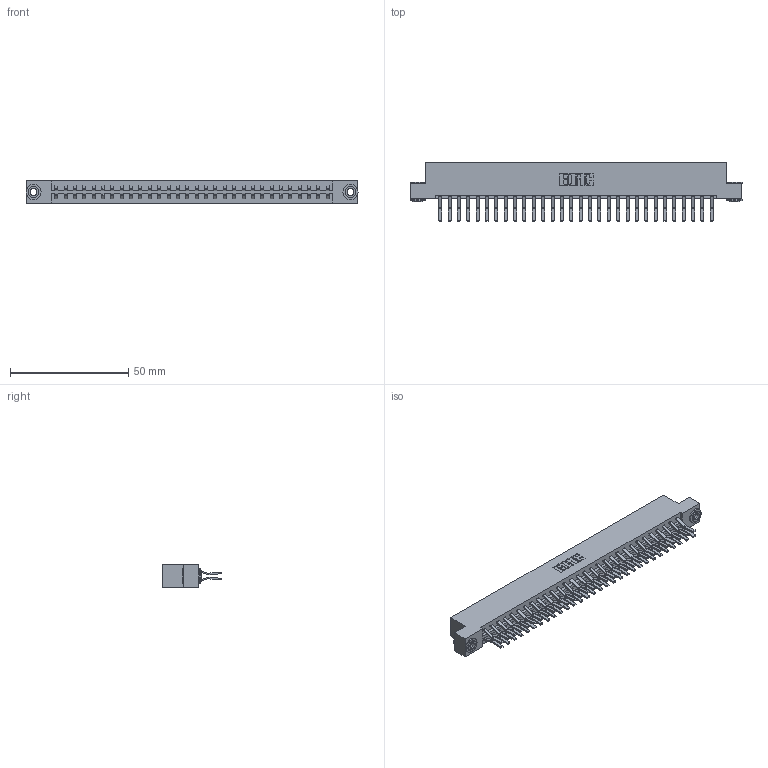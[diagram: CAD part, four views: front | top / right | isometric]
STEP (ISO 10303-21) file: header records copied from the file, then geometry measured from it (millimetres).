
FILE_DESCRIPTION (( 'STEP AP203' ), '1' );
FILE_NAME ('333-060-560-203.STEP', '2018-08-04T07:53:34', ( '' ), ( '' ), 'SwSTEP 2.0', 'SolidWorks 2016', '' );
FILE_SCHEMA (( 'CONFIG_CONTROL_DESIGN' ));
Length unit declared in the file: inch
Products named in the file (4): 345-250-002_345-250-002-102; 333-060-560-203; 333 Part_Flush - .156 Dia - TH; 345-292-001_560 Tail
Assembly tree (63 placements, depth 2):
  333-060-560-203
    333 Part_Flush - .156 Dia - TH
    345-292-001_560 Tail  x60
    345-250-002_345-250-002-102  x2
Bounding box: 140.41 x 24.78 x 9.4 mm (x, y, z)
Volume: 14635.6 mm3; surface area: 18516.8 mm2
Topology: 63 solids, 63 shells, 3392 faces, 10047 edges, 6614 vertices
Faces by surface type: plane 2240, cylinder 1144, cone 8
Entity records: 21590 total; most frequent: CARTESIAN_POINT 3569, ORIENTED_EDGE 3498, DIRECTION 3107, EDGE_CURVE 1749, LINE 1593, VECTOR 1593, VERTEX_POINT 1162, AXIS2_PLACEMENT_3D 757
